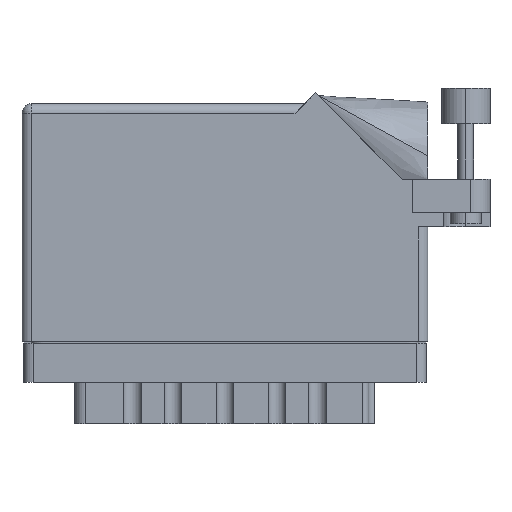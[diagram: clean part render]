
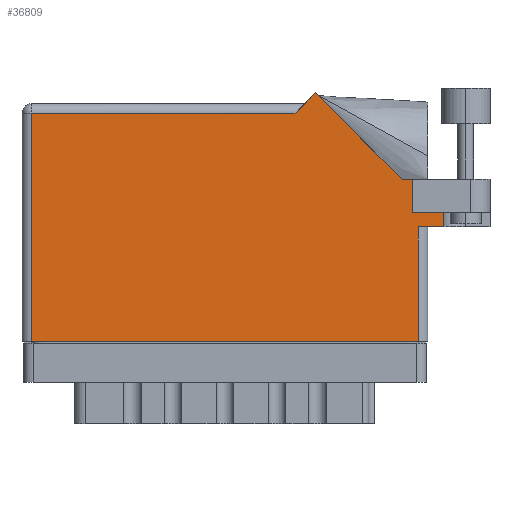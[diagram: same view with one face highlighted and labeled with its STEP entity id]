
A CAD part, front view. The second image highlights one B-rep face of the part: STEP entity #36809.
In plain terms, the highlighted face is planar.
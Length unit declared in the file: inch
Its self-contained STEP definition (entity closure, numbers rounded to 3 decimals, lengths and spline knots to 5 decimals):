
#176 = EDGE_CURVE ( 'NONE', #15159, #9431, #14159, .T. ) ;
#538 = DIRECTION ( 'NONE',  ( 1., 0., 0. ) ) ;
#567 = CARTESIAN_POINT ( 'NONE',  ( 0.062, 0., 0. ) ) ;
#799 = ORIENTED_EDGE ( 'NONE', *, *, #45232, .T. ) ;
#1114 = LINE ( 'NONE', #41616, #14144 ) ;
#1575 = DIRECTION ( 'NONE',  ( -0.707, 0.707, 0. ) ) ;
#1767 = LINE ( 'NONE', #47961, #33613 ) ;
#2045 = ORIENTED_EDGE ( 'NONE', *, *, #176, .T. ) ;
#2048 = EDGE_CURVE ( 'NONE', #12207, #12773, #1767, .T. ) ;
#2443 = CARTESIAN_POINT ( 'NONE',  ( 0., 1.53, 0. ) ) ;
#3306 = VECTOR ( 'NONE', #52303, 39.37008 ) ;
#3320 = VERTEX_POINT ( 'NONE', #50125 ) ;
#5441 = CARTESIAN_POINT ( 'NONE',  ( 2.44642, 1.044, 0. ) ) ;
#5818 = CARTESIAN_POINT ( 'NONE',  ( 2.55, 0., 0. ) ) ;
#6102 = ORIENTED_EDGE ( 'NONE', *, *, #53232, .T. ) ;
#7754 = CARTESIAN_POINT ( 'NONE',  ( 2.55, 0.737, 0. ) ) ;
#8117 = DIRECTION ( 'NONE',  ( 0., 1., 0. ) ) ;
#9431 = VERTEX_POINT ( 'NONE', #53231 ) ;
#9670 = CARTESIAN_POINT ( 'NONE',  ( 1.819, 1.53, 0. ) ) ;
#9962 = DIRECTION ( 'NONE',  ( -1., 0., 0. ) ) ;
#10372 = DIRECTION ( 'NONE',  ( -0.707, -0.707, 0. ) ) ;
#10606 = DIRECTION ( 'NONE',  ( 0., 1., 0. ) ) ;
#10902 = CARTESIAN_POINT ( 'NONE',  ( 3.012, 1.044, 0. ) ) ;
#12124 = EDGE_CURVE ( 'NONE', #22077, #30011, #16625, .T. ) ;
#12207 = VERTEX_POINT ( 'NONE', #45818 ) ;
#12773 = VERTEX_POINT ( 'NONE', #36598 ) ;
#13286 = LINE ( 'NONE', #10902, #52365 ) ;
#13896 = CARTESIAN_POINT ( 'NONE',  ( 1.757, 1.468, 0. ) ) ;
#14144 = VECTOR ( 'NONE', #538, 39.37008 ) ;
#14159 = LINE ( 'NONE', #567, #46069 ) ;
#14646 = DIRECTION ( 'NONE',  ( 0., 0., -1. ) ) ;
#14949 = VERTEX_POINT ( 'NONE', #5441 ) ;
#15138 = CARTESIAN_POINT ( 'NONE',  ( 2.612, 0.737, 0. ) ) ;
#15159 = VERTEX_POINT ( 'NONE', #35730 ) ;
#15394 = EDGE_LOOP ( 'NONE', ( #39471, #24900, #39896, #39753, #23035, #45059, #19525, #799, #6102, #45110, #2045 ) ) ;
#16534 = CARTESIAN_POINT ( 'NONE',  ( 2.7135, 1.16177, 0. ) ) ;
#16625 = LINE ( 'NONE', #7754, #38107 ) ;
#18845 = LINE ( 'NONE', #15138, #3306 ) ;
#19137 = VERTEX_POINT ( 'NONE', #41655 ) ;
#19525 = ORIENTED_EDGE ( 'NONE', *, *, #38878, .T. ) ;
#19617 = EDGE_CURVE ( 'NONE', #12207, #19137, #1114, .T. ) ;
#20487 = VERTEX_POINT ( 'NONE', #13896 ) ;
#22077 = VERTEX_POINT ( 'NONE', #5818 ) ;
#22241 = VECTOR ( 'NONE', #1575, 39.37008 ) ;
#22605 = CARTESIAN_POINT ( 'NONE',  ( 2.44642, 1.044, 0. ) ) ;
#23035 = ORIENTED_EDGE ( 'NONE', *, *, #19617, .F. ) ;
#24577 = EDGE_CURVE ( 'NONE', #19137, #3320, #34007, .T. ) ;
#24900 = ORIENTED_EDGE ( 'NONE', *, *, #12124, .T. ) ;
#26153 = LINE ( 'NONE', #22605, #22241 ) ;
#26787 = EDGE_CURVE ( 'NONE', #30011, #3320, #18845, .T. ) ;
#26937 = CARTESIAN_POINT ( 'NONE',  ( 1.88971, 1.60071, 0. ) ) ;
#26953 = PLANE ( 'NONE',  #43596 ) ;
#30011 = VERTEX_POINT ( 'NONE', #40577 ) ;
#32455 = EDGE_CURVE ( 'NONE', #20487, #15159, #38079, .T. ) ;
#33075 = DIRECTION ( 'NONE',  ( 0., -1., 0. ) ) ;
#33613 = VECTOR ( 'NONE', #10606, 39.37008 ) ;
#33921 = VECTOR ( 'NONE', #39681, 39.37008 ) ;
#34007 = LINE ( 'NONE', #16534, #47162 ) ;
#34851 = VECTOR ( 'NONE', #9962, 39.37008 ) ;
#34965 = VECTOR ( 'NONE', #10372, 39.37008 ) ;
#35179 = CARTESIAN_POINT ( 'NONE',  ( 0., 1.468, 0. ) ) ;
#35730 = CARTESIAN_POINT ( 'NONE',  ( 0.062, 1.468, 0. ) ) ;
#36598 = CARTESIAN_POINT ( 'NONE',  ( 2.512, 1.044, 0. ) ) ;
#36809 = ADVANCED_FACE ( 'NONE', ( #40174 ), #26953, .F. ) ;
#38079 = LINE ( 'NONE', #35179, #34851 ) ;
#38107 = VECTOR ( 'NONE', #8117, 39.37008 ) ;
#38878 = EDGE_CURVE ( 'NONE', #12773, #14949, #13286, .T. ) ;
#39471 = ORIENTED_EDGE ( 'NONE', *, *, #50542, .T. ) ;
#39681 = DIRECTION ( 'NONE',  ( 1., 0., 0. ) ) ;
#39753 = ORIENTED_EDGE ( 'NONE', *, *, #24577, .F. ) ;
#39896 = ORIENTED_EDGE ( 'NONE', *, *, #26787, .T. ) ;
#39982 = VERTEX_POINT ( 'NONE', #26937 ) ;
#40174 = FACE_OUTER_BOUND ( 'NONE', #15394, .T. ) ;
#40577 = CARTESIAN_POINT ( 'NONE',  ( 2.55, 0.737, 0. ) ) ;
#41616 = CARTESIAN_POINT ( 'NONE',  ( 2.512, 0.831, 0. ) ) ;
#41655 = CARTESIAN_POINT ( 'NONE',  ( 2.7135, 0.831, 0. ) ) ;
#42368 = DIRECTION ( 'NONE',  ( 0., -1., 0. ) ) ;
#43596 = AXIS2_PLACEMENT_3D ( 'NONE', #2443, #14646, #52511 ) ;
#44221 = DIRECTION ( 'NONE',  ( -1., 0., 0. ) ) ;
#45039 = LINE ( 'NONE', #47804, #33921 ) ;
#45059 = ORIENTED_EDGE ( 'NONE', *, *, #2048, .T. ) ;
#45110 = ORIENTED_EDGE ( 'NONE', *, *, #32455, .T. ) ;
#45232 = EDGE_CURVE ( 'NONE', #14949, #39982, #26153, .T. ) ;
#45818 = CARTESIAN_POINT ( 'NONE',  ( 2.512, 0.831, 0. ) ) ;
#46069 = VECTOR ( 'NONE', #42368, 39.37008 ) ;
#46108 = LINE ( 'NONE', #9670, #34965 ) ;
#47162 = VECTOR ( 'NONE', #33075, 39.37008 ) ;
#47804 = CARTESIAN_POINT ( 'NONE',  ( 0., 0., 0. ) ) ;
#47961 = CARTESIAN_POINT ( 'NONE',  ( 2.512, 0.831, 0. ) ) ;
#50125 = CARTESIAN_POINT ( 'NONE',  ( 2.7135, 0.737, 0. ) ) ;
#50542 = EDGE_CURVE ( 'NONE', #9431, #22077, #45039, .T. ) ;
#52303 = DIRECTION ( 'NONE',  ( 1., 0., 0. ) ) ;
#52365 = VECTOR ( 'NONE', #44221, 39.37008 ) ;
#52511 = DIRECTION ( 'NONE',  ( -1., 0., 0. ) ) ;
#53231 = CARTESIAN_POINT ( 'NONE',  ( 0.062, 0., 0. ) ) ;
#53232 = EDGE_CURVE ( 'NONE', #39982, #20487, #46108, .T. ) ;
